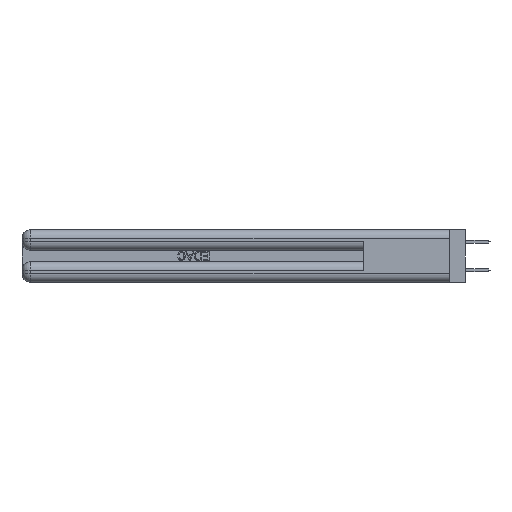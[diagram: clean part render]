
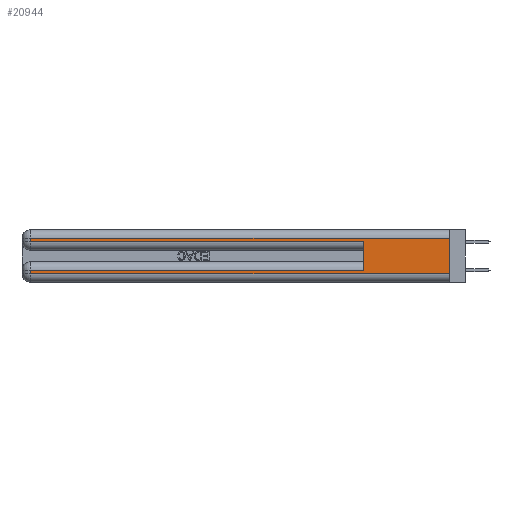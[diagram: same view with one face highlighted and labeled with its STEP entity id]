
A CAD part, left-side view. The second image highlights one B-rep face of the part: STEP entity #20944.
In plain terms, the highlighted planar face has unit normal (-1, 0, 0).
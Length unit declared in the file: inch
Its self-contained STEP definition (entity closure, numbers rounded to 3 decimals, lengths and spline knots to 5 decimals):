
#296 = FACE_OUTER_BOUND ( 'NONE', #22625, .T. ) ;
#1352 = LINE ( 'NONE', #30992, #38843 ) ;
#1948 = VECTOR ( 'NONE', #10232, 39.37008 ) ;
#2670 = ORIENTED_EDGE ( 'NONE', *, *, #16747, .T. ) ;
#2984 = VERTEX_POINT ( 'NONE', #23927 ) ;
#3289 = CARTESIAN_POINT ( 'NONE',  ( 0., 0., 0.37 ) ) ;
#3767 = ORIENTED_EDGE ( 'NONE', *, *, #25099, .T. ) ;
#4084 = VERTEX_POINT ( 'NONE', #43795 ) ;
#4721 = CARTESIAN_POINT ( 'NONE',  ( 0., 0.6, 0.145 ) ) ;
#5238 = LINE ( 'NONE', #38569, #23469 ) ;
#6385 = CARTESIAN_POINT ( 'NONE',  ( 0., 0., 0.285 ) ) ;
#7005 = DIRECTION ( 'NONE',  ( 0., 0., -1. ) ) ;
#9016 = VERTEX_POINT ( 'NONE', #40872 ) ;
#9164 = CARTESIAN_POINT ( 'NONE',  ( 0., 2.94, 0.085 ) ) ;
#10232 = DIRECTION ( 'NONE',  ( 0., 0., -1. ) ) ;
#11002 = VECTOR ( 'NONE', #35447, 39.37008 ) ;
#12142 = LINE ( 'NONE', #6385, #11002 ) ;
#12279 = EDGE_CURVE ( 'NONE', #21610, #2984, #1352, .T. ) ;
#12848 = ORIENTED_EDGE ( 'NONE', *, *, #35908, .F. ) ;
#13381 = CARTESIAN_POINT ( 'NONE',  ( 0., 2.94, 0.31 ) ) ;
#13563 = DIRECTION ( 'NONE',  ( 0., 1., 0. ) ) ;
#14225 = CARTESIAN_POINT ( 'NONE',  ( 0., 0., 0.085 ) ) ;
#16747 = EDGE_CURVE ( 'NONE', #9016, #2984, #20146, .T. ) ;
#16968 = CARTESIAN_POINT ( 'NONE',  ( 0., 0., 0.06 ) ) ;
#17434 = EDGE_CURVE ( 'NONE', #33863, #41721, #12142, .T. ) ;
#18940 = ORIENTED_EDGE ( 'NONE', *, *, #37855, .T. ) ;
#20031 = VERTEX_POINT ( 'NONE', #9164 ) ;
#20146 = LINE ( 'NONE', #16968, #39329 ) ;
#20944 = ADVANCED_FACE ( 'NONE', ( #296 ), #39438, .F. ) ;
#21610 = VERTEX_POINT ( 'NONE', #36321 ) ;
#22625 = EDGE_LOOP ( 'NONE', ( #22723, #18940, #42453, #34076, #12848, #3767, #29485, #2670 ) ) ;
#22723 = ORIENTED_EDGE ( 'NONE', *, *, #12279, .F. ) ;
#22772 = LINE ( 'NONE', #39811, #40790 ) ;
#23469 = VECTOR ( 'NONE', #31503, 39.37008 ) ;
#23927 = CARTESIAN_POINT ( 'NONE',  ( 0., 0., 0.06 ) ) ;
#24690 = LINE ( 'NONE', #14225, #42676 ) ;
#25099 = EDGE_CURVE ( 'NONE', #4084, #20031, #24690, .T. ) ;
#25251 = AXIS2_PLACEMENT_3D ( 'NONE', #3289, #28754, #7005 ) ;
#28754 = DIRECTION ( 'NONE',  ( 1., 0., 0. ) ) ;
#28891 = EDGE_CURVE ( 'NONE', #42914, #33863, #40549, .T. ) ;
#29485 = ORIENTED_EDGE ( 'NONE', *, *, #30631, .T. ) ;
#29742 = LINE ( 'NONE', #4721, #39297 ) ;
#30178 = DIRECTION ( 'NONE',  ( 0., 0., 1. ) ) ;
#30631 = EDGE_CURVE ( 'NONE', #20031, #9016, #5238, .T. ) ;
#30992 = CARTESIAN_POINT ( 'NONE',  ( 0., 0., 0.37 ) ) ;
#31320 = DIRECTION ( 'NONE',  ( 0., 0., -1. ) ) ;
#31503 = DIRECTION ( 'NONE',  ( 0., 0., -1. ) ) ;
#31742 = CARTESIAN_POINT ( 'NONE',  ( 0., 0.6, 0.285 ) ) ;
#33863 = VERTEX_POINT ( 'NONE', #40333 ) ;
#34076 = ORIENTED_EDGE ( 'NONE', *, *, #17434, .T. ) ;
#35447 = DIRECTION ( 'NONE',  ( 0., -1., 0. ) ) ;
#35908 = EDGE_CURVE ( 'NONE', #4084, #41721, #29742, .T. ) ;
#36321 = CARTESIAN_POINT ( 'NONE',  ( 0., 0., 0.31 ) ) ;
#37855 = EDGE_CURVE ( 'NONE', #21610, #42914, #22772, .T. ) ;
#38569 = CARTESIAN_POINT ( 'NONE',  ( 0., 2.94, 0.37 ) ) ;
#38843 = VECTOR ( 'NONE', #31320, 39.37008 ) ;
#39018 = CARTESIAN_POINT ( 'NONE',  ( 0., 2.94, 0.37 ) ) ;
#39297 = VECTOR ( 'NONE', #30178, 39.37008 ) ;
#39329 = VECTOR ( 'NONE', #45738, 39.37008 ) ;
#39438 = PLANE ( 'NONE',  #25251 ) ;
#39811 = CARTESIAN_POINT ( 'NONE',  ( 0., 0., 0.31 ) ) ;
#40333 = CARTESIAN_POINT ( 'NONE',  ( 0., 2.94, 0.285 ) ) ;
#40549 = LINE ( 'NONE', #39018, #1948 ) ;
#40790 = VECTOR ( 'NONE', #13563, 39.37008 ) ;
#40872 = CARTESIAN_POINT ( 'NONE',  ( 0., 2.94, 0.06 ) ) ;
#41721 = VERTEX_POINT ( 'NONE', #31742 ) ;
#42453 = ORIENTED_EDGE ( 'NONE', *, *, #28891, .T. ) ;
#42676 = VECTOR ( 'NONE', #46765, 39.37008 ) ;
#42914 = VERTEX_POINT ( 'NONE', #13381 ) ;
#43795 = CARTESIAN_POINT ( 'NONE',  ( 0., 0.6, 0.085 ) ) ;
#45738 = DIRECTION ( 'NONE',  ( 0., -1., 0. ) ) ;
#46765 = DIRECTION ( 'NONE',  ( 0., 1., 0. ) ) ;
